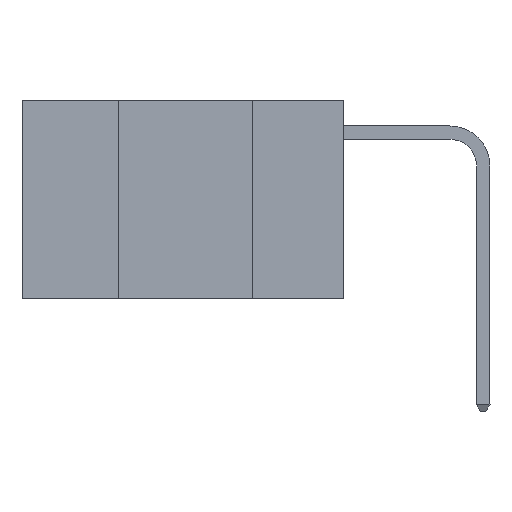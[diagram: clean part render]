
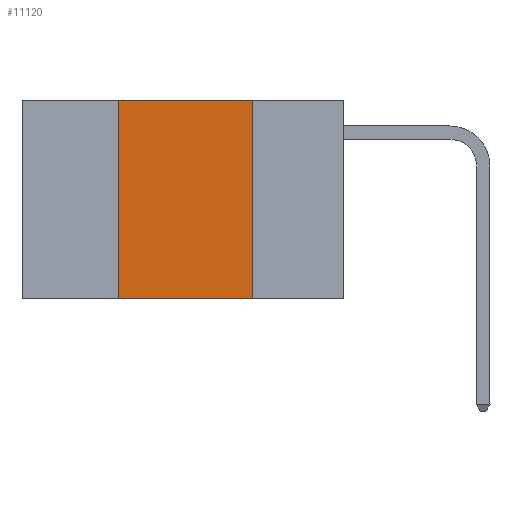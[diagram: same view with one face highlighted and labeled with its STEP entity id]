
A CAD part, left-side view. The second image highlights one B-rep face of the part: STEP entity #11120.
In plain terms, the highlighted planar face has unit normal (-1, 0, 0).
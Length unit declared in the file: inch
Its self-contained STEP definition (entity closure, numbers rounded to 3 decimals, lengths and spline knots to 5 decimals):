
#592 = EDGE_LOOP ( 'NONE', ( #3559, #3964, #1012, #9470 ) ) ;
#1012 = ORIENTED_EDGE ( 'NONE', *, *, #13200, .F. ) ;
#1290 = AXIS2_PLACEMENT_3D ( 'NONE', #1575, #4962, #12952 ) ;
#1481 = DIRECTION ( 'NONE',  ( 0., -1., 0. ) ) ;
#1575 = CARTESIAN_POINT ( 'NONE',  ( 0., 0.6, 0. ) ) ;
#1739 = DIRECTION ( 'NONE',  ( 0., 0., -1. ) ) ;
#2136 = VERTEX_POINT ( 'NONE', #3919 ) ;
#2759 = CARTESIAN_POINT ( 'NONE',  ( 0., 0.6, 0. ) ) ;
#3015 = VERTEX_POINT ( 'NONE', #14564 ) ;
#3559 = ORIENTED_EDGE ( 'NONE', *, *, #10039, .F. ) ;
#3651 = LINE ( 'NONE', #3992, #12060 ) ;
#3919 = CARTESIAN_POINT ( 'NONE',  ( 0., 0.17, -0.37 ) ) ;
#3964 = ORIENTED_EDGE ( 'NONE', *, *, #10637, .F. ) ;
#3992 = CARTESIAN_POINT ( 'NONE',  ( 0., 0.17, 0. ) ) ;
#4149 = VECTOR ( 'NONE', #11897, 39.37008 ) ;
#4962 = DIRECTION ( 'NONE',  ( 1., 0., 0. ) ) ;
#4999 = VECTOR ( 'NONE', #1481, 39.37008 ) ;
#5983 = CARTESIAN_POINT ( 'NONE',  ( 0., 0.6, -0.37 ) ) ;
#6687 = CARTESIAN_POINT ( 'NONE',  ( 0., 0.17, 0. ) ) ;
#7186 = FACE_OUTER_BOUND ( 'NONE', #592, .T. ) ;
#7726 = DIRECTION ( 'NONE',  ( 0., 0., 1. ) ) ;
#8050 = LINE ( 'NONE', #5983, #4999 ) ;
#8114 = PLANE ( 'NONE',  #1290 ) ;
#8447 = VECTOR ( 'NONE', #7726, 39.37008 ) ;
#8801 = LINE ( 'NONE', #14497, #8447 ) ;
#9171 = CARTESIAN_POINT ( 'NONE',  ( 0., 0.42, 0. ) ) ;
#9470 = ORIENTED_EDGE ( 'NONE', *, *, #14410, .T. ) ;
#9854 = LINE ( 'NONE', #2759, #4149 ) ;
#10039 = EDGE_CURVE ( 'NONE', #14171, #2136, #3651, .T. ) ;
#10372 = VERTEX_POINT ( 'NONE', #9171 ) ;
#10637 = EDGE_CURVE ( 'NONE', #10372, #14171, #9854, .T. ) ;
#11120 = ADVANCED_FACE ( 'NONE', ( #7186 ), #8114, .F. ) ;
#11897 = DIRECTION ( 'NONE',  ( 0., -1., 0. ) ) ;
#12060 = VECTOR ( 'NONE', #1739, 39.37008 ) ;
#12952 = DIRECTION ( 'NONE',  ( 0., 0., -1. ) ) ;
#13200 = EDGE_CURVE ( 'NONE', #3015, #10372, #8801, .T. ) ;
#14171 = VERTEX_POINT ( 'NONE', #6687 ) ;
#14410 = EDGE_CURVE ( 'NONE', #3015, #2136, #8050, .T. ) ;
#14497 = CARTESIAN_POINT ( 'NONE',  ( 0., 0.42, 0. ) ) ;
#14564 = CARTESIAN_POINT ( 'NONE',  ( 0., 0.42, -0.37 ) ) ;
